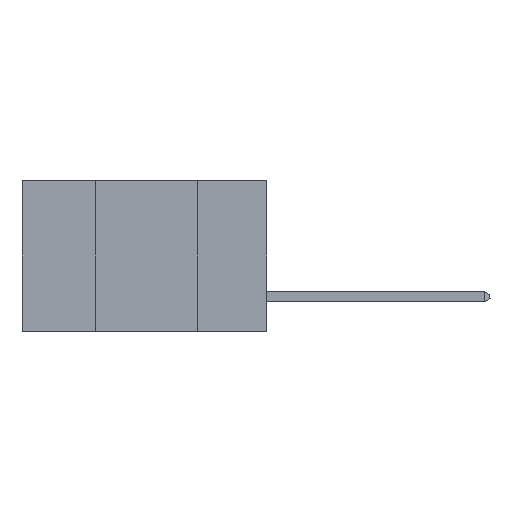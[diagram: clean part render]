
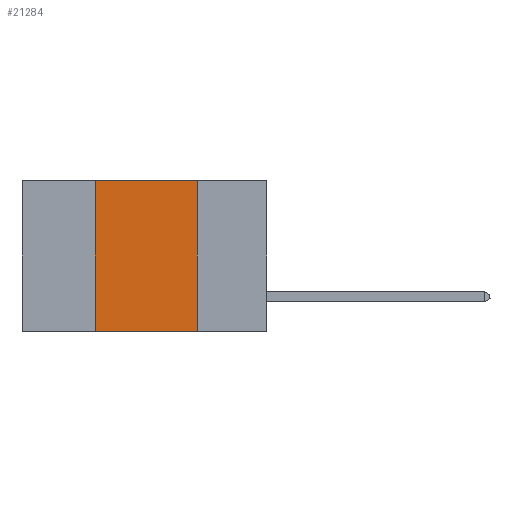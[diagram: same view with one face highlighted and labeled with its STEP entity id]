
A CAD part, left-side view. The second image highlights one B-rep face of the part: STEP entity #21284.
In plain terms, the highlighted planar face has unit normal (-1, 0, 0).
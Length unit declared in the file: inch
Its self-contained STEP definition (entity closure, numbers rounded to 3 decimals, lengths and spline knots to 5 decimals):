
#475 = ORIENTED_EDGE ( 'NONE', *, *, #30851, .F. ) ;
#1029 = CARTESIAN_POINT ( 'NONE',  ( 0., 0.6, -0.37 ) ) ;
#1466 = VERTEX_POINT ( 'NONE', #26169 ) ;
#1833 = VECTOR ( 'NONE', #7690, 39.37008 ) ;
#2198 = EDGE_LOOP ( 'NONE', ( #475, #15175, #32046, #33790 ) ) ;
#3203 = LINE ( 'NONE', #34686, #23643 ) ;
#6521 = VECTOR ( 'NONE', #34672, 39.37008 ) ;
#7452 = CARTESIAN_POINT ( 'NONE',  ( 0., 0.6, 0. ) ) ;
#7690 = DIRECTION ( 'NONE',  ( 0., -1., 0. ) ) ;
#9878 = CARTESIAN_POINT ( 'NONE',  ( 0., 0.17, 0. ) ) ;
#9947 = VERTEX_POINT ( 'NONE', #31697 ) ;
#9987 = EDGE_CURVE ( 'NONE', #1466, #9947, #12173, .T. ) ;
#12173 = LINE ( 'NONE', #1029, #6521 ) ;
#13603 = EDGE_CURVE ( 'NONE', #1466, #30582, #3203, .T. ) ;
#13808 = AXIS2_PLACEMENT_3D ( 'NONE', #14026, #33340, #33455 ) ;
#13891 = VERTEX_POINT ( 'NONE', #9878 ) ;
#14026 = CARTESIAN_POINT ( 'NONE',  ( 0., 0.6, 0. ) ) ;
#15175 = ORIENTED_EDGE ( 'NONE', *, *, #30987, .F. ) ;
#16911 = FACE_OUTER_BOUND ( 'NONE', #2198, .T. ) ;
#17519 = LINE ( 'NONE', #7452, #1833 ) ;
#18784 = DIRECTION ( 'NONE',  ( 0., 0., 1. ) ) ;
#19576 = PLANE ( 'NONE',  #13808 ) ;
#20711 = CARTESIAN_POINT ( 'NONE',  ( 0., 0.17, 0. ) ) ;
#20946 = DIRECTION ( 'NONE',  ( 0., 0., -1. ) ) ;
#21284 = ADVANCED_FACE ( 'NONE', ( #16911 ), #19576, .F. ) ;
#23643 = VECTOR ( 'NONE', #18784, 39.37008 ) ;
#26169 = CARTESIAN_POINT ( 'NONE',  ( 0., 0.42, -0.37 ) ) ;
#27545 = LINE ( 'NONE', #20711, #31900 ) ;
#30513 = CARTESIAN_POINT ( 'NONE',  ( 0., 0.42, 0. ) ) ;
#30582 = VERTEX_POINT ( 'NONE', #30513 ) ;
#30851 = EDGE_CURVE ( 'NONE', #13891, #9947, #27545, .T. ) ;
#30987 = EDGE_CURVE ( 'NONE', #30582, #13891, #17519, .T. ) ;
#31697 = CARTESIAN_POINT ( 'NONE',  ( 0., 0.17, -0.37 ) ) ;
#31900 = VECTOR ( 'NONE', #20946, 39.37008 ) ;
#32046 = ORIENTED_EDGE ( 'NONE', *, *, #13603, .F. ) ;
#33340 = DIRECTION ( 'NONE',  ( 1., 0., 0. ) ) ;
#33455 = DIRECTION ( 'NONE',  ( 0., 0., -1. ) ) ;
#33790 = ORIENTED_EDGE ( 'NONE', *, *, #9987, .T. ) ;
#34672 = DIRECTION ( 'NONE',  ( 0., -1., 0. ) ) ;
#34686 = CARTESIAN_POINT ( 'NONE',  ( 0., 0.42, 0. ) ) ;
